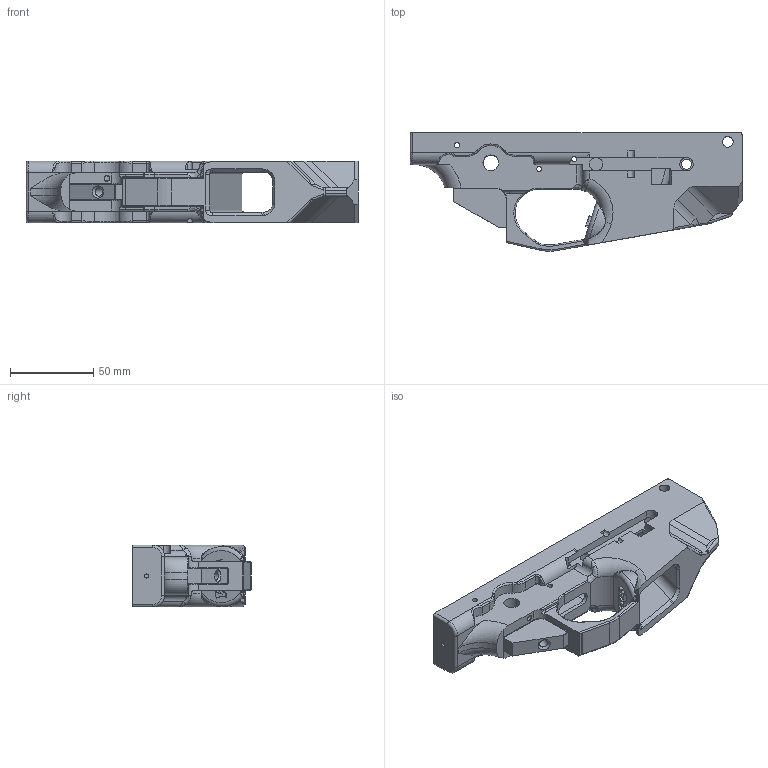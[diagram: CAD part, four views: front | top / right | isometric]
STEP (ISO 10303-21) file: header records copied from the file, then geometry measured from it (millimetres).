
FILE_DESCRIPTION(/* description */ (''),/* implementation_level */ '2;1');
FILE_NAME(/* name */ 'WTF-6MM AIRSOFT VERSION ;).stp',/* time_stamp */ '2020-05-16T00:04:10+03:00',/* author */ (''),/* organization */ (''),/* preprocessor_version */ 'ST-DEVELOPER v15.2',/* originating_system */ 'Autodesk Translator Framework v2.0.0.5431',/* authorisation */ '');
FILE_SCHEMA (('AUTOMOTIVE_DESIGN { 1 0 10303 214 3 1 1 }'));
Length unit declared in the file: centimetre
Bounding box: 199.47 x 71.26 x 37.13 mm (x, y, z)
Volume: 191797.6 mm3; surface area: 54955 mm2
Topology: 1 solids, 1 shells, 643 faces, 1751 edges, 1111 vertices
Faces by surface type: plane 268, bspline 185, cylinder 144, torus 42, sphere 2, cone 2
Full cylindrical faces by diameter (mm): 2.5 x1, 3 x4, 3.175 x3, 3.469 x1, 5.105 x1, 6 x1, 6.4 x2, 8 x1, 9.525 x2, 16.2 x1
Entity records: 30055 total; most frequent: CARTESIAN_POINT 15022, ORIENTED_EDGE 3438, DIRECTION 2603, EDGE_CURVE 1713, VERTEX_POINT 1102, LINE 937, VECTOR 937, AXIS2_PLACEMENT_3D 833
